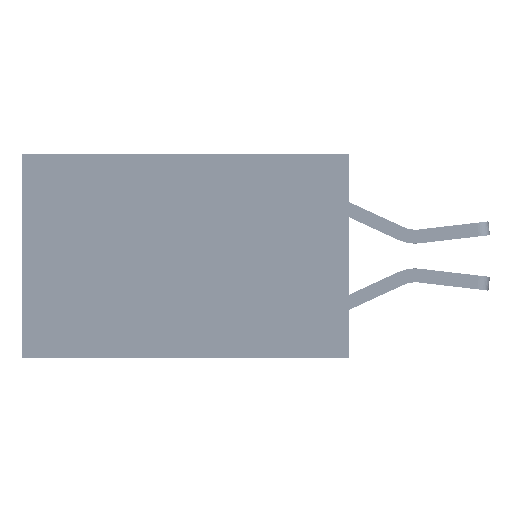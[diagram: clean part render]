
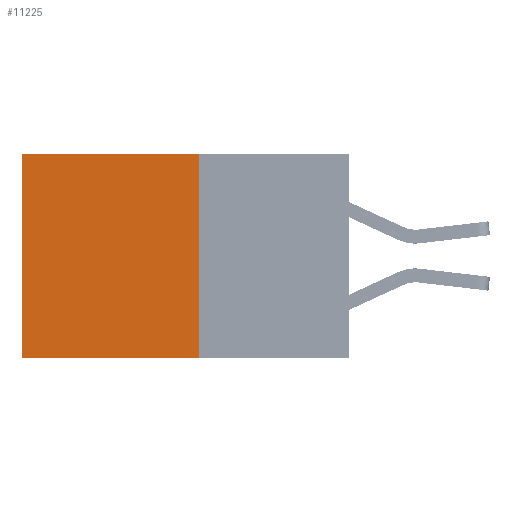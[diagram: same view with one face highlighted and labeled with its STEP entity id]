
A CAD part, left-side view. The second image highlights one B-rep face of the part: STEP entity #11225.
In plain terms, the highlighted planar face has unit normal (-1, 0, 0).
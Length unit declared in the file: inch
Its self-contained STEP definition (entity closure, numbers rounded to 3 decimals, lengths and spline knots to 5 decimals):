
#143 = EDGE_CURVE ( 'NONE', #25299, #7433, #20377, .T. ) ;
#1787 = EDGE_CURVE ( 'NONE', #18119, #24730, #11974, .T. ) ;
#2022 = AXIS2_PLACEMENT_3D ( 'NONE', #28755, #18298, #2186 ) ;
#2057 = PLANE ( 'NONE',  #2022 ) ;
#2163 = CARTESIAN_POINT ( 'NONE',  ( 0.277, 0.27, -0.37 ) ) ;
#2186 = DIRECTION ( 'NONE',  ( 0., 0., -1. ) ) ;
#3512 = ORIENTED_EDGE ( 'NONE', *, *, #143, .F. ) ;
#5881 = ORIENTED_EDGE ( 'NONE', *, *, #1787, .T. ) ;
#7433 = VERTEX_POINT ( 'NONE', #10982 ) ;
#8821 = CARTESIAN_POINT ( 'NONE',  ( 0.277, 0.59, -0.37 ) ) ;
#10982 = CARTESIAN_POINT ( 'NONE',  ( 0.277, 0.59, -0.37 ) ) ;
#11049 = ORIENTED_EDGE ( 'NONE', *, *, #13305, .F. ) ;
#11225 = ADVANCED_FACE ( 'NONE', ( #26860 ), #2057, .F. ) ;
#11813 = DIRECTION ( 'NONE',  ( 0., 1., 0. ) ) ;
#11974 = LINE ( 'NONE', #24374, #18227 ) ;
#12556 = CARTESIAN_POINT ( 'NONE',  ( 0.277, 0.27, 0. ) ) ;
#13073 = LINE ( 'NONE', #2163, #20912 ) ;
#13305 = EDGE_CURVE ( 'NONE', #18119, #25299, #13073, .T. ) ;
#17567 = DIRECTION ( 'NONE',  ( 0., 1., 0. ) ) ;
#17894 = EDGE_LOOP ( 'NONE', ( #34242, #3512, #11049, #5881 ) ) ;
#18119 = VERTEX_POINT ( 'NONE', #12556 ) ;
#18227 = VECTOR ( 'NONE', #11813, 39.37008 ) ;
#18298 = DIRECTION ( 'NONE',  ( 1., 0., 0. ) ) ;
#18978 = CARTESIAN_POINT ( 'NONE',  ( 0.277, 0.59, 0. ) ) ;
#20377 = LINE ( 'NONE', #31234, #33552 ) ;
#20881 = DIRECTION ( 'NONE',  ( 0., 0., -1. ) ) ;
#20912 = VECTOR ( 'NONE', #20881, 39.37008 ) ;
#24374 = CARTESIAN_POINT ( 'NONE',  ( 0.277, 0.27, 0. ) ) ;
#24680 = DIRECTION ( 'NONE',  ( 0., 0., -1. ) ) ;
#24730 = VERTEX_POINT ( 'NONE', #18978 ) ;
#25299 = VERTEX_POINT ( 'NONE', #29077 ) ;
#25539 = EDGE_CURVE ( 'NONE', #24730, #7433, #30070, .T. ) ;
#26860 = FACE_OUTER_BOUND ( 'NONE', #17894, .T. ) ;
#28442 = VECTOR ( 'NONE', #24680, 39.37008 ) ;
#28755 = CARTESIAN_POINT ( 'NONE',  ( 0.277, 0.27, -0.37 ) ) ;
#29077 = CARTESIAN_POINT ( 'NONE',  ( 0.277, 0.27, -0.37 ) ) ;
#30070 = LINE ( 'NONE', #8821, #28442 ) ;
#31234 = CARTESIAN_POINT ( 'NONE',  ( 0.277, 0.27, -0.37 ) ) ;
#33552 = VECTOR ( 'NONE', #17567, 39.37008 ) ;
#34242 = ORIENTED_EDGE ( 'NONE', *, *, #25539, .T. ) ;
